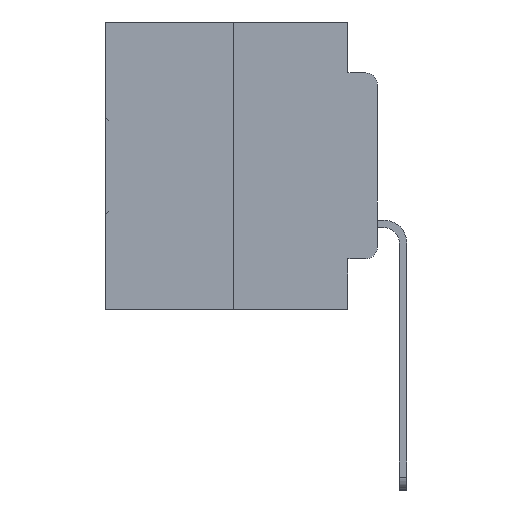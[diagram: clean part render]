
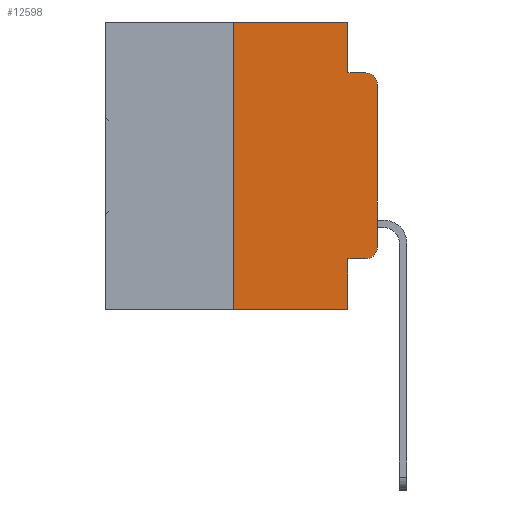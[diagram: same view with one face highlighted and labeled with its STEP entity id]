
A CAD part, left-side view. The second image highlights one B-rep face of the part: STEP entity #12598.
In plain terms, the highlighted planar face has unit normal (-1, 0, 0).
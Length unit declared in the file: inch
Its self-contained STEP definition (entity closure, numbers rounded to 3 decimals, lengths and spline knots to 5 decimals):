
#275 = CARTESIAN_POINT ( 'NONE',  ( 0., 0.02, -0.0885 ) ) ;
#276 = DIRECTION ( 'NONE',  ( -1., 0., 0. ) ) ;
#1093 = DIRECTION ( 'NONE',  ( 0., -1., 0. ) ) ;
#1445 = LINE ( 'NONE', #12850, #21258 ) ;
#1580 = EDGE_CURVE ( 'NONE', #28980, #9616, #7630, .T. ) ;
#1964 = PLANE ( 'NONE',  #2019 ) ;
#2019 = AXIS2_PLACEMENT_3D ( 'NONE', #7500, #25086, #10143 ) ;
#2399 = DIRECTION ( 'NONE',  ( 0., 0., 1. ) ) ;
#2427 = CARTESIAN_POINT ( 'NONE',  ( 0., 0., -0.1085 ) ) ;
#2652 = VERTEX_POINT ( 'NONE', #2427 ) ;
#4759 = VERTEX_POINT ( 'NONE', #22446 ) ;
#7500 = CARTESIAN_POINT ( 'NONE',  ( 0., 0.473, 0. ) ) ;
#7529 = VECTOR ( 'NONE', #18405, 39.37008 ) ;
#7630 = LINE ( 'NONE', #21233, #20220 ) ;
#7948 = EDGE_LOOP ( 'NONE', ( #20467, #20301, #29587, #12165, #25624, #25233, #8178, #22860, #20956, #31301 ) ) ;
#8178 = ORIENTED_EDGE ( 'NONE', *, *, #15713, .T. ) ;
#8641 = EDGE_CURVE ( 'NONE', #28575, #28980, #20354, .T. ) ;
#8921 = CARTESIAN_POINT ( 'NONE',  ( 0., 0.051, -0.0885 ) ) ;
#9100 = CARTESIAN_POINT ( 'NONE',  ( 0., 0.25, 0. ) ) ;
#9616 = VERTEX_POINT ( 'NONE', #275 ) ;
#9674 = CARTESIAN_POINT ( 'NONE',  ( 0., 0.051, -0.4115 ) ) ;
#10095 = CARTESIAN_POINT ( 'NONE',  ( 0., 0.02, -0.1085 ) ) ;
#10143 = DIRECTION ( 'NONE',  ( 0., 0., -1. ) ) ;
#12066 = EDGE_CURVE ( 'NONE', #21714, #26717, #29222, .T. ) ;
#12165 = ORIENTED_EDGE ( 'NONE', *, *, #8641, .F. ) ;
#12596 = DIRECTION ( 'NONE',  ( 0., 0., -1. ) ) ;
#12598 = ADVANCED_FACE ( 'NONE', ( #12851 ), #1964, .F. ) ;
#12656 = CIRCLE ( 'NONE', #13805, 0.02 ) ;
#12660 = DIRECTION ( 'NONE',  ( 0., 0., -1. ) ) ;
#12740 = CARTESIAN_POINT ( 'NONE',  ( 0., 0.051, -0.5 ) ) ;
#12812 = CARTESIAN_POINT ( 'NONE',  ( 0., 0.02, -0.4115 ) ) ;
#12850 = CARTESIAN_POINT ( 'NONE',  ( 0., 0.051, -0.4115 ) ) ;
#12851 = FACE_OUTER_BOUND ( 'NONE', #7948, .T. ) ;
#13326 = VERTEX_POINT ( 'NONE', #9674 ) ;
#13368 = CARTESIAN_POINT ( 'NONE',  ( 0., 0.051, 0. ) ) ;
#13759 = VECTOR ( 'NONE', #31014, 39.37008 ) ;
#13805 = AXIS2_PLACEMENT_3D ( 'NONE', #16070, #276, #18616 ) ;
#14560 = LINE ( 'NONE', #16190, #13759 ) ;
#14767 = EDGE_CURVE ( 'NONE', #13326, #31593, #1445, .T. ) ;
#15291 = CARTESIAN_POINT ( 'NONE',  ( 0., 0.051, 0. ) ) ;
#15441 = DIRECTION ( 'NONE',  ( 0., -1., 0. ) ) ;
#15713 = EDGE_CURVE ( 'NONE', #21714, #15941, #23628, .T. ) ;
#15780 = LINE ( 'NONE', #30863, #28253 ) ;
#15941 = VERTEX_POINT ( 'NONE', #12740 ) ;
#16070 = CARTESIAN_POINT ( 'NONE',  ( 0., 0.02, -0.3915 ) ) ;
#16190 = CARTESIAN_POINT ( 'NONE',  ( 0., 0., 0. ) ) ;
#16334 = DIRECTION ( 'NONE',  ( 0., -1., 0. ) ) ;
#16793 = CARTESIAN_POINT ( 'NONE',  ( 0., 0.473, -0.5 ) ) ;
#16922 = VECTOR ( 'NONE', #1093, 39.37008 ) ;
#18405 = DIRECTION ( 'NONE',  ( 0., 0., -1. ) ) ;
#18616 = DIRECTION ( 'NONE',  ( 0., 0., -1. ) ) ;
#20220 = VECTOR ( 'NONE', #16334, 39.37008 ) ;
#20301 = ORIENTED_EDGE ( 'NONE', *, *, #27466, .T. ) ;
#20354 = LINE ( 'NONE', #25111, #25446 ) ;
#20358 = EDGE_CURVE ( 'NONE', #26717, #28575, #15780, .T. ) ;
#20467 = ORIENTED_EDGE ( 'NONE', *, *, #22540, .T. ) ;
#20905 = LINE ( 'NONE', #13368, #7529 ) ;
#20956 = ORIENTED_EDGE ( 'NONE', *, *, #14767, .T. ) ;
#21233 = CARTESIAN_POINT ( 'NONE',  ( 0., 0.051, -0.0885 ) ) ;
#21258 = VECTOR ( 'NONE', #15441, 39.37008 ) ;
#21714 = VERTEX_POINT ( 'NONE', #32017 ) ;
#22446 = CARTESIAN_POINT ( 'NONE',  ( 0., 0., -0.3915 ) ) ;
#22540 = EDGE_CURVE ( 'NONE', #4759, #2652, #14560, .T. ) ;
#22707 = VECTOR ( 'NONE', #2399, 39.37008 ) ;
#22860 = ORIENTED_EDGE ( 'NONE', *, *, #27064, .F. ) ;
#23628 = LINE ( 'NONE', #16793, #16922 ) ;
#24072 = CIRCLE ( 'NONE', #24125, 0.02 ) ;
#24125 = AXIS2_PLACEMENT_3D ( 'NONE', #10095, #27500, #12596 ) ;
#25086 = DIRECTION ( 'NONE',  ( 1., 0., 0. ) ) ;
#25111 = CARTESIAN_POINT ( 'NONE',  ( 0., 0.051, 0. ) ) ;
#25233 = ORIENTED_EDGE ( 'NONE', *, *, #12066, .F. ) ;
#25446 = VECTOR ( 'NONE', #12660, 39.37008 ) ;
#25624 = ORIENTED_EDGE ( 'NONE', *, *, #20358, .F. ) ;
#26048 = DIRECTION ( 'NONE',  ( 0., -1., 0. ) ) ;
#26717 = VERTEX_POINT ( 'NONE', #9100 ) ;
#27064 = EDGE_CURVE ( 'NONE', #13326, #15941, #20905, .T. ) ;
#27466 = EDGE_CURVE ( 'NONE', #2652, #9616, #24072, .T. ) ;
#27500 = DIRECTION ( 'NONE',  ( -1., 0., 0. ) ) ;
#28138 = EDGE_CURVE ( 'NONE', #31593, #4759, #12656, .T. ) ;
#28253 = VECTOR ( 'NONE', #26048, 39.37008 ) ;
#28575 = VERTEX_POINT ( 'NONE', #15291 ) ;
#28980 = VERTEX_POINT ( 'NONE', #8921 ) ;
#29222 = LINE ( 'NONE', #32665, #22707 ) ;
#29587 = ORIENTED_EDGE ( 'NONE', *, *, #1580, .F. ) ;
#30863 = CARTESIAN_POINT ( 'NONE',  ( 0., 0.473, 0. ) ) ;
#31014 = DIRECTION ( 'NONE',  ( 0., 0., 1. ) ) ;
#31301 = ORIENTED_EDGE ( 'NONE', *, *, #28138, .T. ) ;
#31593 = VERTEX_POINT ( 'NONE', #12812 ) ;
#32017 = CARTESIAN_POINT ( 'NONE',  ( 0., 0.25, -0.5 ) ) ;
#32665 = CARTESIAN_POINT ( 'NONE',  ( 0., 0.25, 0. ) ) ;
